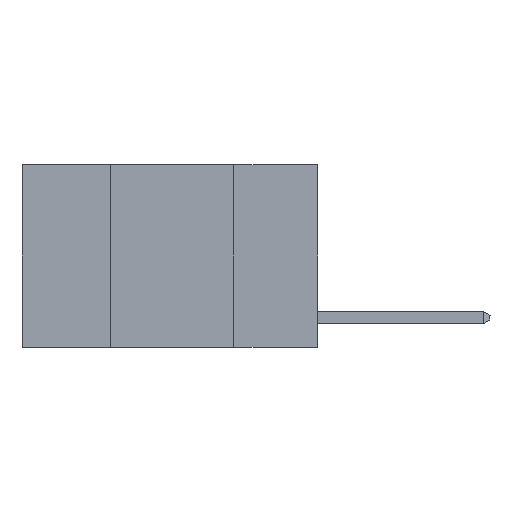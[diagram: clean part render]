
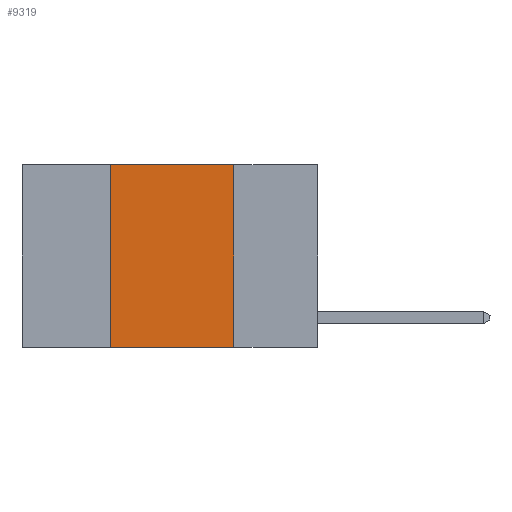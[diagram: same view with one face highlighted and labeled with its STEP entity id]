
A CAD part, left-side view. The second image highlights one B-rep face of the part: STEP entity #9319.
In plain terms, the highlighted planar face has unit normal (-1, 0, 0).
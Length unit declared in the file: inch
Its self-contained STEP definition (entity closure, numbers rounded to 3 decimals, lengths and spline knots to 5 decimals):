
#196 = VECTOR ( 'NONE', #12638, 39.37008 ) ;
#227 = DIRECTION ( 'NONE',  ( 0., 0., 1. ) ) ;
#268 = CARTESIAN_POINT ( 'NONE',  ( 0., 0.42, -0.37 ) ) ;
#427 = VERTEX_POINT ( 'NONE', #5597 ) ;
#536 = ORIENTED_EDGE ( 'NONE', *, *, #12392, .F. ) ;
#1671 = LINE ( 'NONE', #7602, #196 ) ;
#2219 = FACE_OUTER_BOUND ( 'NONE', #2230, .T. ) ;
#2230 = EDGE_LOOP ( 'NONE', ( #10227, #6723, #536, #12154 ) ) ;
#2866 = EDGE_CURVE ( 'NONE', #10348, #427, #2928, .T. ) ;
#2928 = LINE ( 'NONE', #11824, #3591 ) ;
#2988 = CARTESIAN_POINT ( 'NONE',  ( 0., 0.17, 0. ) ) ;
#3239 = CARTESIAN_POINT ( 'NONE',  ( 0., 0.42, 0. ) ) ;
#3292 = DIRECTION ( 'NONE',  ( 0., 0., -1. ) ) ;
#3591 = VECTOR ( 'NONE', #3292, 39.37008 ) ;
#3686 = VERTEX_POINT ( 'NONE', #268 ) ;
#4089 = VERTEX_POINT ( 'NONE', #5448 ) ;
#4367 = DIRECTION ( 'NONE',  ( 0., -1., 0. ) ) ;
#5448 = CARTESIAN_POINT ( 'NONE',  ( 0., 0.42, 0. ) ) ;
#5597 = CARTESIAN_POINT ( 'NONE',  ( 0., 0.17, -0.37 ) ) ;
#5953 = AXIS2_PLACEMENT_3D ( 'NONE', #12529, #8370, #7127 ) ;
#6080 = PLANE ( 'NONE',  #5953 ) ;
#6458 = CARTESIAN_POINT ( 'NONE',  ( 0., 0.6, -0.37 ) ) ;
#6723 = ORIENTED_EDGE ( 'NONE', *, *, #12468, .F. ) ;
#7127 = DIRECTION ( 'NONE',  ( 0., 0., -1. ) ) ;
#7145 = EDGE_CURVE ( 'NONE', #3686, #427, #11948, .T. ) ;
#7191 = LINE ( 'NONE', #3239, #13094 ) ;
#7602 = CARTESIAN_POINT ( 'NONE',  ( 0., 0.6, 0. ) ) ;
#8188 = VECTOR ( 'NONE', #4367, 39.37008 ) ;
#8370 = DIRECTION ( 'NONE',  ( 1., 0., 0. ) ) ;
#9319 = ADVANCED_FACE ( 'NONE', ( #2219 ), #6080, .F. ) ;
#10227 = ORIENTED_EDGE ( 'NONE', *, *, #2866, .F. ) ;
#10348 = VERTEX_POINT ( 'NONE', #2988 ) ;
#11824 = CARTESIAN_POINT ( 'NONE',  ( 0., 0.17, 0. ) ) ;
#11948 = LINE ( 'NONE', #6458, #8188 ) ;
#12154 = ORIENTED_EDGE ( 'NONE', *, *, #7145, .T. ) ;
#12392 = EDGE_CURVE ( 'NONE', #3686, #4089, #7191, .T. ) ;
#12468 = EDGE_CURVE ( 'NONE', #4089, #10348, #1671, .T. ) ;
#12529 = CARTESIAN_POINT ( 'NONE',  ( 0., 0.6, 0. ) ) ;
#12638 = DIRECTION ( 'NONE',  ( 0., -1., 0. ) ) ;
#13094 = VECTOR ( 'NONE', #227, 39.37008 ) ;
